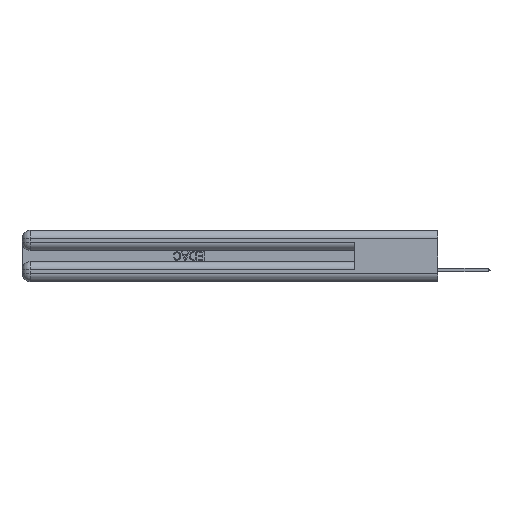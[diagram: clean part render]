
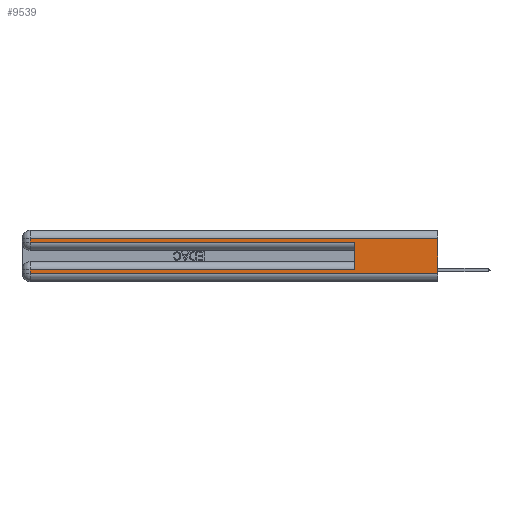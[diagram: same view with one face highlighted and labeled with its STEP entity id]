
A CAD part, left-side view. The second image highlights one B-rep face of the part: STEP entity #9539.
In plain terms, the highlighted planar face has unit normal (-1, 0, 0).
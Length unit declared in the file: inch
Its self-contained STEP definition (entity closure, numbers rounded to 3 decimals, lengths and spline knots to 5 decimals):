
#173 = CARTESIAN_POINT ( 'NONE',  ( 0., 0.6, 0.145 ) ) ;
#1058 = CARTESIAN_POINT ( 'NONE',  ( 0., 0., 0.37 ) ) ;
#3306 = CARTESIAN_POINT ( 'NONE',  ( 0., 0., 0.37 ) ) ;
#5713 = VECTOR ( 'NONE', #39556, 39.37008 ) ;
#6067 = VERTEX_POINT ( 'NONE', #53897 ) ;
#6884 = LINE ( 'NONE', #18397, #51175 ) ;
#7161 = LINE ( 'NONE', #47713, #5713 ) ;
#8477 = LINE ( 'NONE', #10620, #27368 ) ;
#9539 = ADVANCED_FACE ( 'NONE', ( #41352 ), #36591, .F. ) ;
#9591 = VERTEX_POINT ( 'NONE', #28607 ) ;
#9652 = VERTEX_POINT ( 'NONE', #30121 ) ;
#9802 = VERTEX_POINT ( 'NONE', #50522 ) ;
#10620 = CARTESIAN_POINT ( 'NONE',  ( 0., 2.94, 0.37 ) ) ;
#11206 = ORIENTED_EDGE ( 'NONE', *, *, #42230, .T. ) ;
#11631 = EDGE_CURVE ( 'NONE', #9802, #14615, #15083, .T. ) ;
#12150 = EDGE_LOOP ( 'NONE', ( #51962, #17730, #11206, #30495, #30525, #25136, #41472, #45795 ) ) ;
#12349 = EDGE_CURVE ( 'NONE', #16948, #9591, #7161, .T. ) ;
#13701 = VECTOR ( 'NONE', #42973, 39.37008 ) ;
#14615 = VERTEX_POINT ( 'NONE', #19138 ) ;
#14658 = DIRECTION ( 'NONE',  ( 0., 0., -1. ) ) ;
#15083 = LINE ( 'NONE', #21466, #35272 ) ;
#15197 = EDGE_CURVE ( 'NONE', #38253, #9652, #45501, .T. ) ;
#16948 = VERTEX_POINT ( 'NONE', #40287 ) ;
#17730 = ORIENTED_EDGE ( 'NONE', *, *, #11631, .T. ) ;
#18397 = CARTESIAN_POINT ( 'NONE',  ( 0., 2.94, 0.37 ) ) ;
#18431 = CARTESIAN_POINT ( 'NONE',  ( 0., 0., 0.085 ) ) ;
#19138 = CARTESIAN_POINT ( 'NONE',  ( 0., 2.94, 0.31 ) ) ;
#21466 = CARTESIAN_POINT ( 'NONE',  ( 0., 0., 0.31 ) ) ;
#22648 = DIRECTION ( 'NONE',  ( 0., 1., 0. ) ) ;
#23623 = DIRECTION ( 'NONE',  ( 0., -1., 0. ) ) ;
#25136 = ORIENTED_EDGE ( 'NONE', *, *, #15197, .T. ) ;
#25865 = VECTOR ( 'NONE', #23623, 39.37008 ) ;
#27248 = CARTESIAN_POINT ( 'NONE',  ( 0., 0., 0.06 ) ) ;
#27368 = VECTOR ( 'NONE', #14658, 39.37008 ) ;
#28491 = CARTESIAN_POINT ( 'NONE',  ( 0., 2.94, 0.06 ) ) ;
#28576 = LINE ( 'NONE', #27248, #25865 ) ;
#28607 = CARTESIAN_POINT ( 'NONE',  ( 0., 0.6, 0.285 ) ) ;
#29210 = CARTESIAN_POINT ( 'NONE',  ( 0., 0.6, 0.085 ) ) ;
#29481 = EDGE_CURVE ( 'NONE', #47877, #6067, #28576, .T. ) ;
#30121 = CARTESIAN_POINT ( 'NONE',  ( 0., 2.94, 0.085 ) ) ;
#30495 = ORIENTED_EDGE ( 'NONE', *, *, #12349, .T. ) ;
#30525 = ORIENTED_EDGE ( 'NONE', *, *, #46718, .F. ) ;
#31822 = VECTOR ( 'NONE', #22648, 39.37008 ) ;
#35272 = VECTOR ( 'NONE', #46217, 39.37008 ) ;
#36591 = PLANE ( 'NONE',  #38247 ) ;
#37164 = DIRECTION ( 'NONE',  ( 1., 0., 0. ) ) ;
#38247 = AXIS2_PLACEMENT_3D ( 'NONE', #3306, #37164, #45145 ) ;
#38253 = VERTEX_POINT ( 'NONE', #29210 ) ;
#39556 = DIRECTION ( 'NONE',  ( 0., -1., 0. ) ) ;
#40287 = CARTESIAN_POINT ( 'NONE',  ( 0., 2.94, 0.285 ) ) ;
#41022 = EDGE_CURVE ( 'NONE', #9802, #6067, #50864, .T. ) ;
#41352 = FACE_OUTER_BOUND ( 'NONE', #12150, .T. ) ;
#41472 = ORIENTED_EDGE ( 'NONE', *, *, #44194, .T. ) ;
#42230 = EDGE_CURVE ( 'NONE', #14615, #16948, #8477, .T. ) ;
#42973 = DIRECTION ( 'NONE',  ( 0., 0., -1. ) ) ;
#44194 = EDGE_CURVE ( 'NONE', #9652, #47877, #6884, .T. ) ;
#45145 = DIRECTION ( 'NONE',  ( 0., 0., -1. ) ) ;
#45499 = DIRECTION ( 'NONE',  ( 0., 0., 1. ) ) ;
#45501 = LINE ( 'NONE', #18431, #31822 ) ;
#45795 = ORIENTED_EDGE ( 'NONE', *, *, #29481, .T. ) ;
#46183 = VECTOR ( 'NONE', #45499, 39.37008 ) ;
#46217 = DIRECTION ( 'NONE',  ( 0., 1., 0. ) ) ;
#46718 = EDGE_CURVE ( 'NONE', #38253, #9591, #46755, .T. ) ;
#46755 = LINE ( 'NONE', #173, #46183 ) ;
#47713 = CARTESIAN_POINT ( 'NONE',  ( 0., 0., 0.285 ) ) ;
#47877 = VERTEX_POINT ( 'NONE', #28491 ) ;
#50522 = CARTESIAN_POINT ( 'NONE',  ( 0., 0., 0.31 ) ) ;
#50864 = LINE ( 'NONE', #1058, #13701 ) ;
#51019 = DIRECTION ( 'NONE',  ( 0., 0., -1. ) ) ;
#51175 = VECTOR ( 'NONE', #51019, 39.37008 ) ;
#51962 = ORIENTED_EDGE ( 'NONE', *, *, #41022, .F. ) ;
#53897 = CARTESIAN_POINT ( 'NONE',  ( 0., 0., 0.06 ) ) ;
